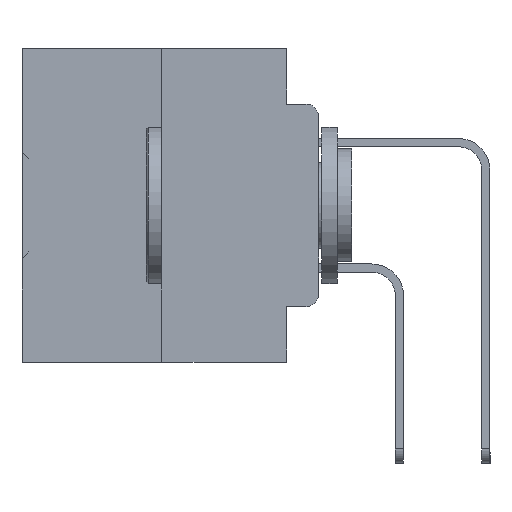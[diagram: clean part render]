
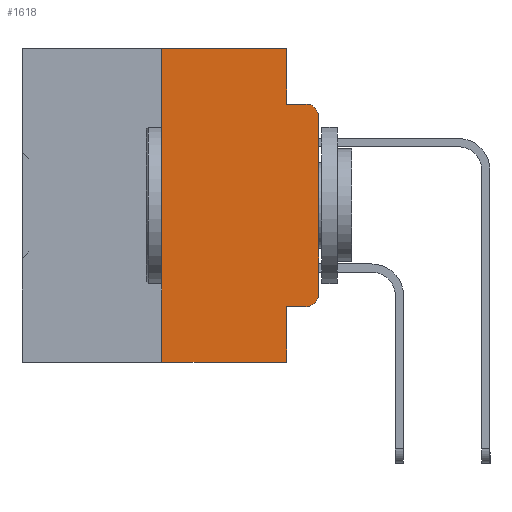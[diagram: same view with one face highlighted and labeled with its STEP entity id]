
A CAD part, left-side view. The second image highlights one B-rep face of the part: STEP entity #1618.
In plain terms, the highlighted planar face has unit normal (-1, 0, 0).
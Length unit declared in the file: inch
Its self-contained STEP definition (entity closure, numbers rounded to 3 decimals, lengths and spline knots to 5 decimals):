
#31 = DIRECTION ( 'NONE',  ( 0., 0., -1. ) ) ;
#945 = EDGE_LOOP ( 'NONE', ( #26183, #34300, #36213, #22846, #9053, #17488, #33847, #12010, #7587, #2203 ) ) ;
#1468 = EDGE_CURVE ( 'NONE', #9794, #22791, #20254, .T. ) ;
#1618 = ADVANCED_FACE ( 'NONE', ( #31761 ), #33289, .F. ) ;
#1851 = VERTEX_POINT ( 'NONE', #22866 ) ;
#2203 = ORIENTED_EDGE ( 'NONE', *, *, #39706, .T. ) ;
#2591 = LINE ( 'NONE', #35962, #8960 ) ;
#2704 = DIRECTION ( 'NONE',  ( -1., 0., 0. ) ) ;
#3391 = CARTESIAN_POINT ( 'NONE',  ( 0., 0., 0. ) ) ;
#3603 = EDGE_CURVE ( 'NONE', #9794, #1851, #2591, .T. ) ;
#3675 = VECTOR ( 'NONE', #29646, 39.37008 ) ;
#4376 = VERTEX_POINT ( 'NONE', #39655 ) ;
#4573 = DIRECTION ( 'NONE',  ( 0., -1., 0. ) ) ;
#5394 = LINE ( 'NONE', #35526, #20168 ) ;
#5703 = AXIS2_PLACEMENT_3D ( 'NONE', #36364, #17990, #39425 ) ;
#6314 = VERTEX_POINT ( 'NONE', #34191 ) ;
#7506 = VECTOR ( 'NONE', #28379, 39.37008 ) ;
#7587 = ORIENTED_EDGE ( 'NONE', *, *, #1468, .T. ) ;
#7697 = CARTESIAN_POINT ( 'NONE',  ( 0., 0.473, -0.5 ) ) ;
#8169 = VERTEX_POINT ( 'NONE', #8934 ) ;
#8791 = CARTESIAN_POINT ( 'NONE',  ( 0., 0.25, -0.5 ) ) ;
#8934 = CARTESIAN_POINT ( 'NONE',  ( 0., 0.051, -0.0885 ) ) ;
#8960 = VECTOR ( 'NONE', #17726, 39.37008 ) ;
#9053 = ORIENTED_EDGE ( 'NONE', *, *, #12882, .F. ) ;
#9794 = VERTEX_POINT ( 'NONE', #29330 ) ;
#9876 = EDGE_CURVE ( 'NONE', #12483, #4376, #26315, .T. ) ;
#10887 = DIRECTION ( 'NONE',  ( 0., -1., 0. ) ) ;
#11715 = CARTESIAN_POINT ( 'NONE',  ( 0., 0.02, -0.1085 ) ) ;
#11838 = VECTOR ( 'NONE', #10887, 39.37008 ) ;
#12002 = EDGE_CURVE ( 'NONE', #6314, #8169, #39976, .T. ) ;
#12010 = ORIENTED_EDGE ( 'NONE', *, *, #3603, .F. ) ;
#12483 = VERTEX_POINT ( 'NONE', #8791 ) ;
#12882 = EDGE_CURVE ( 'NONE', #4376, #6314, #23676, .T. ) ;
#14099 = CARTESIAN_POINT ( 'NONE',  ( 0., 0.051, -0.4115 ) ) ;
#14142 = EDGE_CURVE ( 'NONE', #8169, #27905, #5394, .T. ) ;
#14433 = VECTOR ( 'NONE', #31, 39.37008 ) ;
#14928 = DIRECTION ( 'NONE',  ( 0., 0., -1. ) ) ;
#15071 = AXIS2_PLACEMENT_3D ( 'NONE', #11715, #33429, #14928 ) ;
#15365 = VECTOR ( 'NONE', #20635, 39.37008 ) ;
#16047 = CIRCLE ( 'NONE', #15071, 0.02 ) ;
#16728 = CARTESIAN_POINT ( 'NONE',  ( 0., 0.02, -0.0885 ) ) ;
#17475 = DIRECTION ( 'NONE',  ( 0., 0., 1. ) ) ;
#17488 = ORIENTED_EDGE ( 'NONE', *, *, #9876, .F. ) ;
#17726 = DIRECTION ( 'NONE',  ( 0., 0., -1. ) ) ;
#17990 = DIRECTION ( 'NONE',  ( 1., 0., 0. ) ) ;
#20168 = VECTOR ( 'NONE', #4573, 39.37008 ) ;
#20254 = LINE ( 'NONE', #14099, #11838 ) ;
#20406 = VERTEX_POINT ( 'NONE', #38610 ) ;
#20635 = DIRECTION ( 'NONE',  ( 0., -1., 0. ) ) ;
#21560 = CARTESIAN_POINT ( 'NONE',  ( 0., 0.02, -0.3915 ) ) ;
#22073 = CARTESIAN_POINT ( 'NONE',  ( 0., 0.051, 0. ) ) ;
#22582 = EDGE_CURVE ( 'NONE', #20406, #27905, #16047, .T. ) ;
#22791 = VERTEX_POINT ( 'NONE', #31150 ) ;
#22846 = ORIENTED_EDGE ( 'NONE', *, *, #12002, .F. ) ;
#22865 = AXIS2_PLACEMENT_3D ( 'NONE', #21560, #2704, #24663 ) ;
#22866 = CARTESIAN_POINT ( 'NONE',  ( 0., 0.051, -0.5 ) ) ;
#23105 = EDGE_CURVE ( 'NONE', #12483, #1851, #28571, .T. ) ;
#23676 = LINE ( 'NONE', #26819, #15365 ) ;
#24649 = EDGE_CURVE ( 'NONE', #31146, #20406, #25201, .T. ) ;
#24663 = DIRECTION ( 'NONE',  ( 0., 0., -1. ) ) ;
#25201 = LINE ( 'NONE', #3391, #7506 ) ;
#26183 = ORIENTED_EDGE ( 'NONE', *, *, #24649, .T. ) ;
#26315 = LINE ( 'NONE', #38929, #33473 ) ;
#26517 = CIRCLE ( 'NONE', #22865, 0.02 ) ;
#26819 = CARTESIAN_POINT ( 'NONE',  ( 0., 0.473, 0. ) ) ;
#27905 = VERTEX_POINT ( 'NONE', #16728 ) ;
#28379 = DIRECTION ( 'NONE',  ( 0., 0., 1. ) ) ;
#28571 = LINE ( 'NONE', #7697, #3675 ) ;
#29330 = CARTESIAN_POINT ( 'NONE',  ( 0., 0.051, -0.4115 ) ) ;
#29646 = DIRECTION ( 'NONE',  ( 0., -1., 0. ) ) ;
#31146 = VERTEX_POINT ( 'NONE', #32524 ) ;
#31150 = CARTESIAN_POINT ( 'NONE',  ( 0., 0.02, -0.4115 ) ) ;
#31761 = FACE_OUTER_BOUND ( 'NONE', #945, .T. ) ;
#32524 = CARTESIAN_POINT ( 'NONE',  ( 0., 0., -0.3915 ) ) ;
#33289 = PLANE ( 'NONE',  #5703 ) ;
#33429 = DIRECTION ( 'NONE',  ( -1., 0., 0. ) ) ;
#33473 = VECTOR ( 'NONE', #17475, 39.37008 ) ;
#33847 = ORIENTED_EDGE ( 'NONE', *, *, #23105, .T. ) ;
#34191 = CARTESIAN_POINT ( 'NONE',  ( 0., 0.051, 0. ) ) ;
#34300 = ORIENTED_EDGE ( 'NONE', *, *, #22582, .T. ) ;
#35526 = CARTESIAN_POINT ( 'NONE',  ( 0., 0.051, -0.0885 ) ) ;
#35962 = CARTESIAN_POINT ( 'NONE',  ( 0., 0.051, 0. ) ) ;
#36213 = ORIENTED_EDGE ( 'NONE', *, *, #14142, .F. ) ;
#36364 = CARTESIAN_POINT ( 'NONE',  ( 0., 0.473, 0. ) ) ;
#38610 = CARTESIAN_POINT ( 'NONE',  ( 0., 0., -0.1085 ) ) ;
#38929 = CARTESIAN_POINT ( 'NONE',  ( 0., 0.25, 0. ) ) ;
#39425 = DIRECTION ( 'NONE',  ( 0., 0., -1. ) ) ;
#39655 = CARTESIAN_POINT ( 'NONE',  ( 0., 0.25, 0. ) ) ;
#39706 = EDGE_CURVE ( 'NONE', #22791, #31146, #26517, .T. ) ;
#39976 = LINE ( 'NONE', #22073, #14433 ) ;
